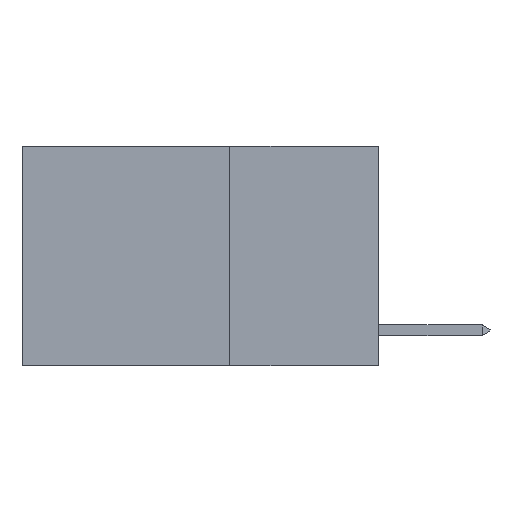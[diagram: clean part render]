
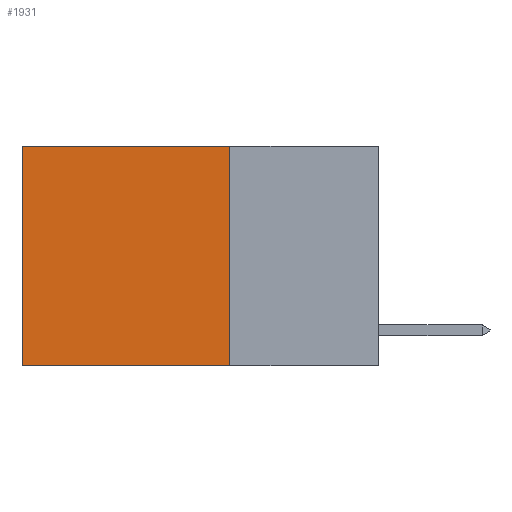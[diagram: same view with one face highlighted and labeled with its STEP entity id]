
A CAD part, left-side view. The second image highlights one B-rep face of the part: STEP entity #1931.
In plain terms, the highlighted planar face has unit normal (-1, 0, 0).
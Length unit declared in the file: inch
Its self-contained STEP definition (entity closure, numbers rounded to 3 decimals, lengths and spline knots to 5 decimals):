
#99 = VERTEX_POINT ( 'NONE', #5297 ) ;
#178 = ORIENTED_EDGE ( 'NONE', *, *, #3187, .T. ) ;
#435 = ORIENTED_EDGE ( 'NONE', *, *, #2903, .F. ) ;
#783 = DIRECTION ( 'NONE',  ( 0., 1., 0. ) ) ;
#820 = CARTESIAN_POINT ( 'NONE',  ( 0.2625, 0.6, -0.37 ) ) ;
#1673 = VERTEX_POINT ( 'NONE', #820 ) ;
#1760 = VERTEX_POINT ( 'NONE', #11651 ) ;
#1931 = ADVANCED_FACE ( 'NONE', ( #8596 ), #2421, .F. ) ;
#2326 = EDGE_CURVE ( 'NONE', #1760, #2348, #5553, .T. ) ;
#2348 = VERTEX_POINT ( 'NONE', #3492 ) ;
#2421 = PLANE ( 'NONE',  #11941 ) ;
#2620 = ORIENTED_EDGE ( 'NONE', *, *, #11368, .F. ) ;
#2903 = EDGE_CURVE ( 'NONE', #99, #1673, #7912, .T. ) ;
#3187 = EDGE_CURVE ( 'NONE', #2348, #1673, #5446, .T. ) ;
#3469 = VECTOR ( 'NONE', #783, 39.37008 ) ;
#3492 = CARTESIAN_POINT ( 'NONE',  ( 0.2625, 0.6, 0. ) ) ;
#4017 = VECTOR ( 'NONE', #7592, 39.37008 ) ;
#4038 = CARTESIAN_POINT ( 'NONE',  ( 0.2625, 0.25, 0. ) ) ;
#4094 = CARTESIAN_POINT ( 'NONE',  ( 0.2625, 0.6, 0. ) ) ;
#4470 = CARTESIAN_POINT ( 'NONE',  ( 0.2625, 0.25, 0. ) ) ;
#4823 = DIRECTION ( 'NONE',  ( 0., 0., -1. ) ) ;
#5043 = ORIENTED_EDGE ( 'NONE', *, *, #2326, .T. ) ;
#5297 = CARTESIAN_POINT ( 'NONE',  ( 0.2625, 0.25, -0.37 ) ) ;
#5433 = DIRECTION ( 'NONE',  ( 0., 0., -1. ) ) ;
#5446 = LINE ( 'NONE', #4094, #7275 ) ;
#5553 = LINE ( 'NONE', #4470, #11275 ) ;
#7275 = VECTOR ( 'NONE', #5433, 39.37008 ) ;
#7304 = EDGE_LOOP ( 'NONE', ( #178, #435, #2620, #5043 ) ) ;
#7592 = DIRECTION ( 'NONE',  ( 0., 0., -1. ) ) ;
#7912 = LINE ( 'NONE', #14734, #3469 ) ;
#8596 = FACE_OUTER_BOUND ( 'NONE', #7304, .T. ) ;
#10521 = DIRECTION ( 'NONE',  ( 0., 1., 0. ) ) ;
#10703 = CARTESIAN_POINT ( 'NONE',  ( 0.2625, 0.25, 0. ) ) ;
#11275 = VECTOR ( 'NONE', #10521, 39.37008 ) ;
#11368 = EDGE_CURVE ( 'NONE', #1760, #99, #13470, .T. ) ;
#11651 = CARTESIAN_POINT ( 'NONE',  ( 0.2625, 0.25, 0. ) ) ;
#11906 = DIRECTION ( 'NONE',  ( 1., 0., 0. ) ) ;
#11941 = AXIS2_PLACEMENT_3D ( 'NONE', #10703, #11906, #4823 ) ;
#13470 = LINE ( 'NONE', #4038, #4017 ) ;
#14734 = CARTESIAN_POINT ( 'NONE',  ( 0.2625, 0.25, -0.37 ) ) ;
